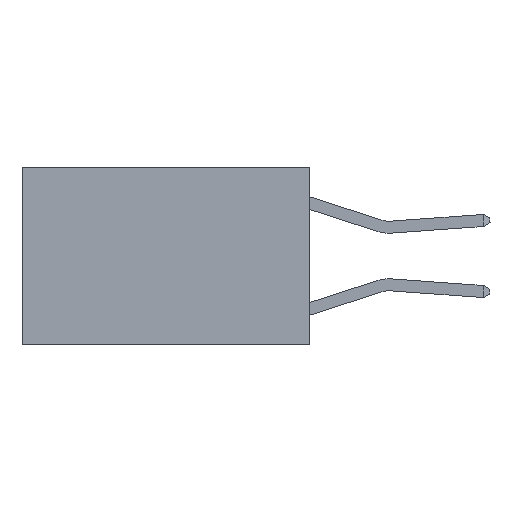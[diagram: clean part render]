
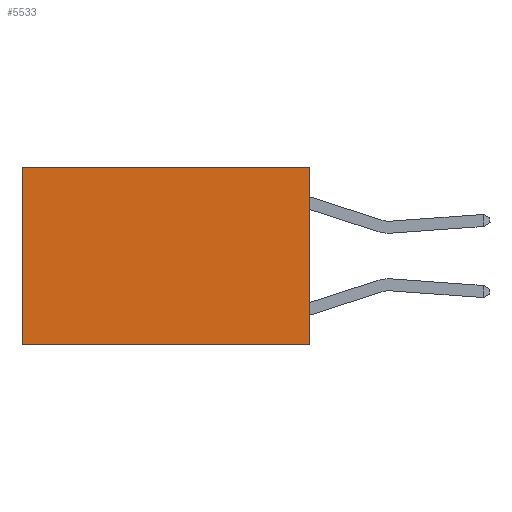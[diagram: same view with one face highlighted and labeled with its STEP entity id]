
A CAD part, left-side view. The second image highlights one B-rep face of the part: STEP entity #5533.
In plain terms, the highlighted planar face has unit normal (-1, 0, 0).
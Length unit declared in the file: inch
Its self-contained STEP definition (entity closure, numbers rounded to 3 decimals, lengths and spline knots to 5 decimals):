
#725 = DIRECTION ( 'NONE',  ( 1., 0., 0. ) ) ;
#1251 = LINE ( 'NONE', #11689, #5751 ) ;
#1463 = ORIENTED_EDGE ( 'NONE', *, *, #2156, .F. ) ;
#1528 = VERTEX_POINT ( 'NONE', #2761 ) ;
#2156 = EDGE_CURVE ( 'NONE', #1528, #7026, #9153, .T. ) ;
#2270 = AXIS2_PLACEMENT_3D ( 'NONE', #6111, #725, #7037 ) ;
#2496 = PLANE ( 'NONE',  #2270 ) ;
#2515 = VECTOR ( 'NONE', #6394, 39.37008 ) ;
#2551 = EDGE_CURVE ( 'NONE', #8284, #7026, #3072, .T. ) ;
#2680 = DIRECTION ( 'NONE',  ( 0., 1., 0. ) ) ;
#2761 = CARTESIAN_POINT ( 'NONE',  ( 0.2625, 0., -0.37 ) ) ;
#3072 = LINE ( 'NONE', #4313, #9995 ) ;
#3267 = CARTESIAN_POINT ( 'NONE',  ( 0.2625, 0., 0. ) ) ;
#3418 = ORIENTED_EDGE ( 'NONE', *, *, #4462, .F. ) ;
#3485 = EDGE_LOOP ( 'NONE', ( #4900, #1463, #3418, #9100 ) ) ;
#4056 = CARTESIAN_POINT ( 'NONE',  ( 0.2625, 0.6, -0.37 ) ) ;
#4313 = CARTESIAN_POINT ( 'NONE',  ( 0.2625, 0.6, 0. ) ) ;
#4412 = EDGE_CURVE ( 'NONE', #10612, #8284, #1251, .T. ) ;
#4462 = EDGE_CURVE ( 'NONE', #10612, #1528, #7884, .T. ) ;
#4561 = CARTESIAN_POINT ( 'NONE',  ( 0.2625, 0., 0. ) ) ;
#4670 = CARTESIAN_POINT ( 'NONE',  ( 0.2625, 0., -0.37 ) ) ;
#4900 = ORIENTED_EDGE ( 'NONE', *, *, #2551, .T. ) ;
#4917 = VECTOR ( 'NONE', #5574, 39.37008 ) ;
#5178 = DIRECTION ( 'NONE',  ( 0., 0., -1. ) ) ;
#5533 = ADVANCED_FACE ( 'NONE', ( #7711 ), #2496, .F. ) ;
#5574 = DIRECTION ( 'NONE',  ( 0., 1., 0. ) ) ;
#5751 = VECTOR ( 'NONE', #2680, 39.37008 ) ;
#6111 = CARTESIAN_POINT ( 'NONE',  ( 0.2625, 0., 0. ) ) ;
#6394 = DIRECTION ( 'NONE',  ( 0., 0., -1. ) ) ;
#7026 = VERTEX_POINT ( 'NONE', #4056 ) ;
#7037 = DIRECTION ( 'NONE',  ( 0., 0., -1. ) ) ;
#7711 = FACE_OUTER_BOUND ( 'NONE', #3485, .T. ) ;
#7884 = LINE ( 'NONE', #4561, #2515 ) ;
#8284 = VERTEX_POINT ( 'NONE', #10077 ) ;
#9100 = ORIENTED_EDGE ( 'NONE', *, *, #4412, .T. ) ;
#9153 = LINE ( 'NONE', #4670, #4917 ) ;
#9995 = VECTOR ( 'NONE', #5178, 39.37008 ) ;
#10077 = CARTESIAN_POINT ( 'NONE',  ( 0.2625, 0.6, 0. ) ) ;
#10612 = VERTEX_POINT ( 'NONE', #3267 ) ;
#11689 = CARTESIAN_POINT ( 'NONE',  ( 0.2625, 0., 0. ) ) ;
